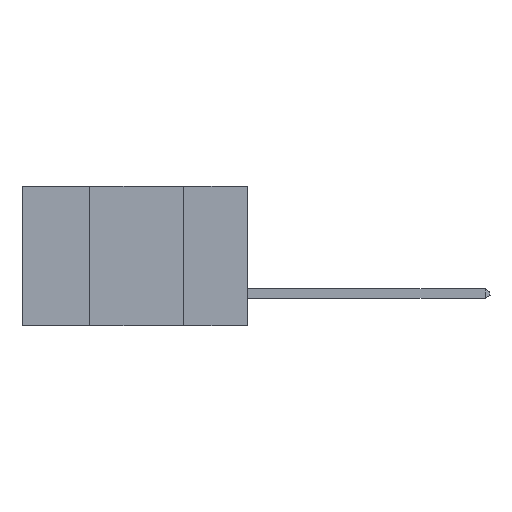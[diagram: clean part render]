
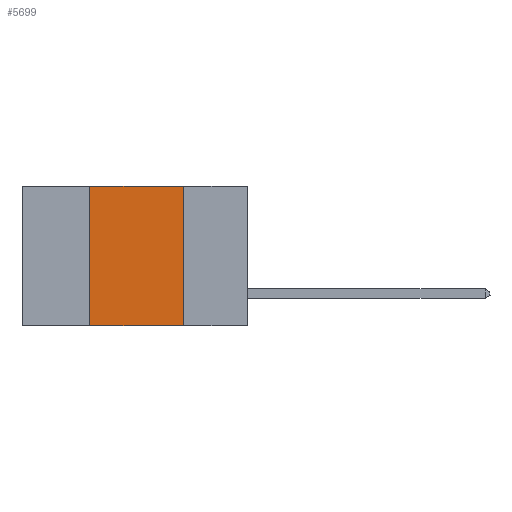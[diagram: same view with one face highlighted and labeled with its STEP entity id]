
A CAD part, left-side view. The second image highlights one B-rep face of the part: STEP entity #5699.
In plain terms, the highlighted planar face has unit normal (-1, 0, 0).
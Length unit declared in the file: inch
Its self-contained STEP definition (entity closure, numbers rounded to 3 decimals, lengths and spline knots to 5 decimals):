
#385 = VECTOR ( 'NONE', #8147, 39.37008 ) ;
#784 = CARTESIAN_POINT ( 'NONE',  ( 0., 0.6, -0.37 ) ) ;
#941 = LINE ( 'NONE', #2073, #5474 ) ;
#1359 = EDGE_CURVE ( 'NONE', #11612, #7578, #4100, .T. ) ;
#1570 = VERTEX_POINT ( 'NONE', #3955 ) ;
#1672 = FACE_OUTER_BOUND ( 'NONE', #6161, .T. ) ;
#2073 = CARTESIAN_POINT ( 'NONE',  ( 0., 0.6, 0. ) ) ;
#2129 = EDGE_CURVE ( 'NONE', #1570, #2851, #7968, .T. ) ;
#2540 = DIRECTION ( 'NONE',  ( 0., 0., -1. ) ) ;
#2630 = CARTESIAN_POINT ( 'NONE',  ( 0., 0.17, 0. ) ) ;
#2851 = VERTEX_POINT ( 'NONE', #9672 ) ;
#3015 = ORIENTED_EDGE ( 'NONE', *, *, #5151, .T. ) ;
#3397 = LINE ( 'NONE', #784, #10316 ) ;
#3955 = CARTESIAN_POINT ( 'NONE',  ( 0., 0.17, 0. ) ) ;
#3968 = DIRECTION ( 'NONE',  ( 0., -1., 0. ) ) ;
#4024 = ORIENTED_EDGE ( 'NONE', *, *, #9143, .F. ) ;
#4100 = LINE ( 'NONE', #6295, #385 ) ;
#4322 = DIRECTION ( 'NONE',  ( 0., 0., -1. ) ) ;
#4418 = CARTESIAN_POINT ( 'NONE',  ( 0., 0.42, 0. ) ) ;
#5151 = EDGE_CURVE ( 'NONE', #11612, #2851, #3397, .T. ) ;
#5474 = VECTOR ( 'NONE', #3968, 39.37008 ) ;
#5699 = ADVANCED_FACE ( 'NONE', ( #1672 ), #6805, .F. ) ;
#6161 = EDGE_LOOP ( 'NONE', ( #11215, #4024, #8440, #3015 ) ) ;
#6230 = DIRECTION ( 'NONE',  ( 0., -1., 0. ) ) ;
#6295 = CARTESIAN_POINT ( 'NONE',  ( 0., 0.42, 0. ) ) ;
#6687 = VECTOR ( 'NONE', #4322, 39.37008 ) ;
#6805 = PLANE ( 'NONE',  #7464 ) ;
#7034 = DIRECTION ( 'NONE',  ( 1., 0., 0. ) ) ;
#7464 = AXIS2_PLACEMENT_3D ( 'NONE', #11502, #7034, #2540 ) ;
#7578 = VERTEX_POINT ( 'NONE', #4418 ) ;
#7968 = LINE ( 'NONE', #2630, #6687 ) ;
#8147 = DIRECTION ( 'NONE',  ( 0., 0., 1. ) ) ;
#8440 = ORIENTED_EDGE ( 'NONE', *, *, #1359, .F. ) ;
#9130 = CARTESIAN_POINT ( 'NONE',  ( 0., 0.42, -0.37 ) ) ;
#9143 = EDGE_CURVE ( 'NONE', #7578, #1570, #941, .T. ) ;
#9672 = CARTESIAN_POINT ( 'NONE',  ( 0., 0.17, -0.37 ) ) ;
#10316 = VECTOR ( 'NONE', #6230, 39.37008 ) ;
#11215 = ORIENTED_EDGE ( 'NONE', *, *, #2129, .F. ) ;
#11502 = CARTESIAN_POINT ( 'NONE',  ( 0., 0.6, 0. ) ) ;
#11612 = VERTEX_POINT ( 'NONE', #9130 ) ;
